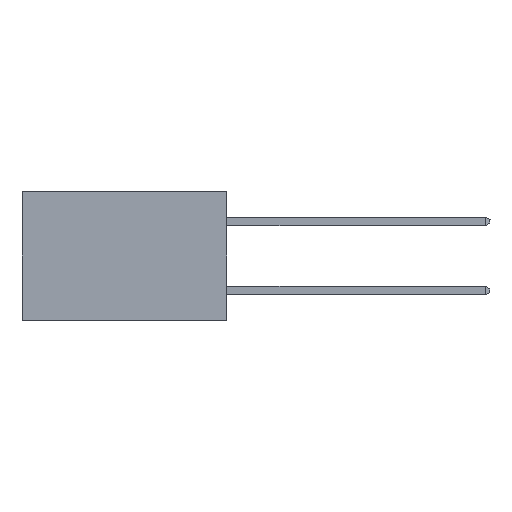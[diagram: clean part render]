
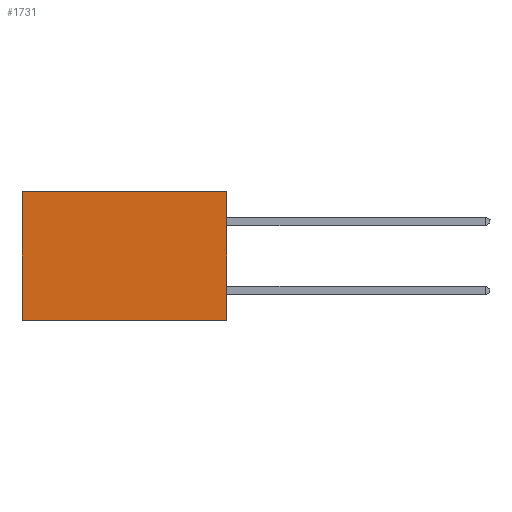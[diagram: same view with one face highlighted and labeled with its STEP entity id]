
A CAD part, left-side view. The second image highlights one B-rep face of the part: STEP entity #1731.
In plain terms, the highlighted planar face has unit normal (-1, 0, 0).
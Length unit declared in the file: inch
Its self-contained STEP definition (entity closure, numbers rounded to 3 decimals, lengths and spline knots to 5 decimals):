
#1672 = ORIENTED_EDGE ( 'NONE', *, *, #13275, .F. ) ;
#1731 = ADVANCED_FACE ( 'NONE', ( #6946 ), #7932, .F. ) ;
#2253 = LINE ( 'NONE', #8111, #5691 ) ;
#3305 = CARTESIAN_POINT ( 'NONE',  ( 0.277, 0., 0. ) ) ;
#4051 = CARTESIAN_POINT ( 'NONE',  ( 0.277, 0., 0. ) ) ;
#4832 = CARTESIAN_POINT ( 'NONE',  ( 0.277, 0.59, 0. ) ) ;
#5530 = DIRECTION ( 'NONE',  ( 0., 0., -1. ) ) ;
#5691 = VECTOR ( 'NONE', #9530, 39.37008 ) ;
#5914 = LINE ( 'NONE', #12771, #17442 ) ;
#6929 = ORIENTED_EDGE ( 'NONE', *, *, #10373, .F. ) ;
#6946 = FACE_OUTER_BOUND ( 'NONE', #13330, .T. ) ;
#6994 = VERTEX_POINT ( 'NONE', #11211 ) ;
#7405 = ORIENTED_EDGE ( 'NONE', *, *, #13436, .T. ) ;
#7578 = CARTESIAN_POINT ( 'NONE',  ( 0.277, 0., -0.37 ) ) ;
#7919 = DIRECTION ( 'NONE',  ( 1., 0., 0. ) ) ;
#7932 = PLANE ( 'NONE',  #14441 ) ;
#8111 = CARTESIAN_POINT ( 'NONE',  ( 0.277, 0., -0.37 ) ) ;
#8609 = DIRECTION ( 'NONE',  ( 0., 0., -1. ) ) ;
#8984 = VERTEX_POINT ( 'NONE', #14119 ) ;
#9530 = DIRECTION ( 'NONE',  ( 0., 1., 0. ) ) ;
#9666 = VECTOR ( 'NONE', #14257, 39.37008 ) ;
#10373 = EDGE_CURVE ( 'NONE', #10560, #6994, #13225, .T. ) ;
#10560 = VERTEX_POINT ( 'NONE', #3305 ) ;
#11211 = CARTESIAN_POINT ( 'NONE',  ( 0.277, 0., -0.37 ) ) ;
#12540 = VERTEX_POINT ( 'NONE', #4832 ) ;
#12759 = VECTOR ( 'NONE', #17390, 39.37008 ) ;
#12771 = CARTESIAN_POINT ( 'NONE',  ( 0.277, 0.59, -0.37 ) ) ;
#13225 = LINE ( 'NONE', #14514, #12759 ) ;
#13275 = EDGE_CURVE ( 'NONE', #6994, #8984, #2253, .T. ) ;
#13330 = EDGE_LOOP ( 'NONE', ( #7405, #1672, #6929, #18200 ) ) ;
#13436 = EDGE_CURVE ( 'NONE', #12540, #8984, #5914, .T. ) ;
#13553 = LINE ( 'NONE', #4051, #9666 ) ;
#14119 = CARTESIAN_POINT ( 'NONE',  ( 0.277, 0.59, -0.37 ) ) ;
#14257 = DIRECTION ( 'NONE',  ( 0., 1., 0. ) ) ;
#14441 = AXIS2_PLACEMENT_3D ( 'NONE', #7578, #7919, #8609 ) ;
#14514 = CARTESIAN_POINT ( 'NONE',  ( 0.277, 0., -0.37 ) ) ;
#15683 = EDGE_CURVE ( 'NONE', #10560, #12540, #13553, .T. ) ;
#17390 = DIRECTION ( 'NONE',  ( 0., 0., -1. ) ) ;
#17442 = VECTOR ( 'NONE', #5530, 39.37008 ) ;
#18200 = ORIENTED_EDGE ( 'NONE', *, *, #15683, .T. ) ;
